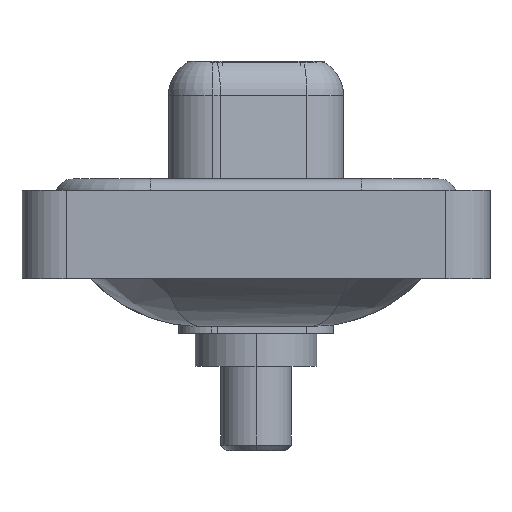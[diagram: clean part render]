
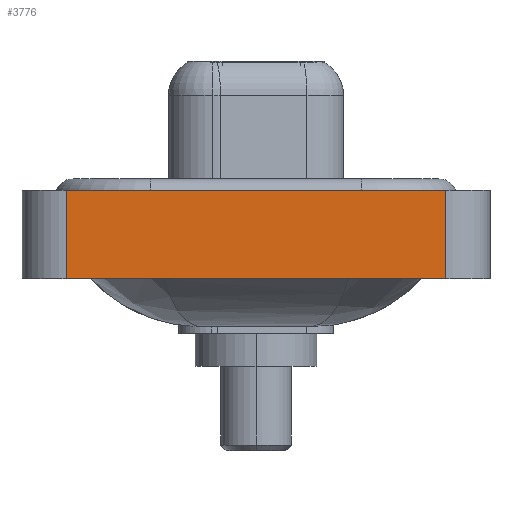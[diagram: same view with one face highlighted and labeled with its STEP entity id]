
A CAD part, left-side view. The second image highlights one B-rep face of the part: STEP entity #3776.
In plain terms, the highlighted planar face has unit normal (-1, 0, 0).
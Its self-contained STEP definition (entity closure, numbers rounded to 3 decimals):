
#832 = CARTESIAN_POINT ( 'NONE',  ( -7.25, -8.55, -3.6 ) ) ;
#1123 = AXIS2_PLACEMENT_3D ( 'NONE', #832, #8578, #9762 ) ;
#1471 = CARTESIAN_POINT ( 'NONE',  ( -7.25, -8.55, 0.4 ) ) ;
#1954 = ORIENTED_EDGE ( 'NONE', *, *, #16309, .T. ) ;
#2555 = VERTEX_POINT ( 'NONE', #11521 ) ;
#2742 = EDGE_CURVE ( 'NONE', #3872, #8389, #14184, .T. ) ;
#3356 = FACE_OUTER_BOUND ( 'NONE', #4213, .T. ) ;
#3776 = ADVANCED_FACE ( 'NONE', ( #3356 ), #16312, .T. ) ;
#3872 = VERTEX_POINT ( 'NONE', #10860 ) ;
#4213 = EDGE_LOOP ( 'NONE', ( #5378, #9225, #16038, #1954 ) ) ;
#5179 = CARTESIAN_POINT ( 'NONE',  ( -7.25, 8.55, 0.4 ) ) ;
#5187 = DIRECTION ( 'NONE',  ( 0., -1., 0. ) ) ;
#5378 = ORIENTED_EDGE ( 'NONE', *, *, #10905, .T. ) ;
#6813 = VECTOR ( 'NONE', #9776, 1000. ) ;
#7152 = LINE ( 'NONE', #12294, #6813 ) ;
#8389 = VERTEX_POINT ( 'NONE', #5179 ) ;
#8578 = DIRECTION ( 'NONE',  ( -1., 0., 0. ) ) ;
#8688 = DIRECTION ( 'NONE',  ( 0., 0., 1. ) ) ;
#9145 = LINE ( 'NONE', #1471, #15026 ) ;
#9225 = ORIENTED_EDGE ( 'NONE', *, *, #10135, .F. ) ;
#9762 = DIRECTION ( 'NONE',  ( 0., 0., 1. ) ) ;
#9776 = DIRECTION ( 'NONE',  ( 0., -1., 0. ) ) ;
#9879 = CARTESIAN_POINT ( 'NONE',  ( -7.25, -8.55, -3.6 ) ) ;
#10135 = EDGE_CURVE ( 'NONE', #8389, #2555, #9145, .T. ) ;
#10466 = VECTOR ( 'NONE', #11842, 1000. ) ;
#10860 = CARTESIAN_POINT ( 'NONE',  ( -7.25, 8.55, -3.6 ) ) ;
#10905 = EDGE_CURVE ( 'NONE', #12348, #2555, #12567, .T. ) ;
#11244 = VECTOR ( 'NONE', #8688, 1000. ) ;
#11521 = CARTESIAN_POINT ( 'NONE',  ( -7.25, -8.55, 0.4 ) ) ;
#11842 = DIRECTION ( 'NONE',  ( 0., 0., 1. ) ) ;
#11923 = CARTESIAN_POINT ( 'NONE',  ( -7.25, 8.55, -3.6 ) ) ;
#12294 = CARTESIAN_POINT ( 'NONE',  ( -7.25, -8.55, -3.6 ) ) ;
#12348 = VERTEX_POINT ( 'NONE', #12810 ) ;
#12567 = LINE ( 'NONE', #9879, #11244 ) ;
#12810 = CARTESIAN_POINT ( 'NONE',  ( -7.25, -8.55, -3.6 ) ) ;
#14184 = LINE ( 'NONE', #11923, #10466 ) ;
#15026 = VECTOR ( 'NONE', #5187, 1000. ) ;
#16038 = ORIENTED_EDGE ( 'NONE', *, *, #2742, .F. ) ;
#16309 = EDGE_CURVE ( 'NONE', #3872, #12348, #7152, .T. ) ;
#16312 = PLANE ( 'NONE',  #1123 ) ;
